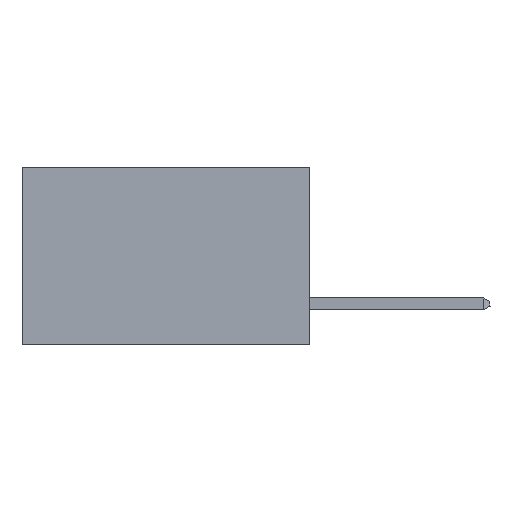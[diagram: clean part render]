
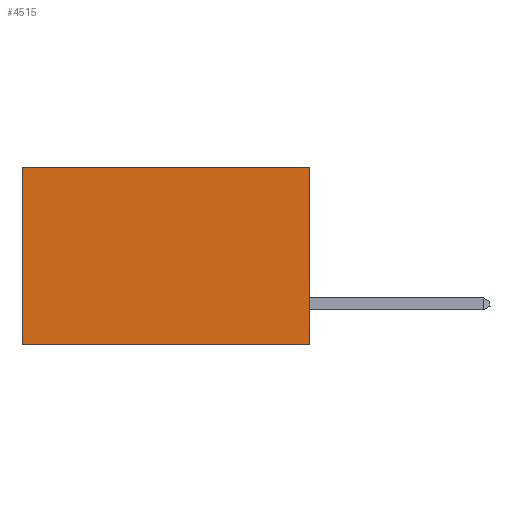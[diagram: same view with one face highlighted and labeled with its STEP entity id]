
A CAD part, left-side view. The second image highlights one B-rep face of the part: STEP entity #4515.
In plain terms, the highlighted planar face has unit normal (-1, 0, 0).
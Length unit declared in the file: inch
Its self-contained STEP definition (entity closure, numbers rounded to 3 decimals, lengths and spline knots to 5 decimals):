
#1781 = CARTESIAN_POINT ( 'NONE',  ( 0.2875, 0., -0.37 ) ) ;
#1880 = FACE_OUTER_BOUND ( 'NONE', #12481, .T. ) ;
#2175 = PLANE ( 'NONE',  #12967 ) ;
#2364 = EDGE_CURVE ( 'NONE', #7530, #5329, #20781, .T. ) ;
#2672 = EDGE_CURVE ( 'NONE', #15979, #6745, #7477, .T. ) ;
#4515 = ADVANCED_FACE ( 'NONE', ( #1880 ), #2175, .F. ) ;
#5237 = CARTESIAN_POINT ( 'NONE',  ( 0.2875, 0., 0. ) ) ;
#5238 = EDGE_CURVE ( 'NONE', #5329, #6745, #22425, .T. ) ;
#5329 = VERTEX_POINT ( 'NONE', #9780 ) ;
#5501 = VECTOR ( 'NONE', #18746, 39.37008 ) ;
#6745 = VERTEX_POINT ( 'NONE', #16134 ) ;
#7477 = LINE ( 'NONE', #1781, #21686 ) ;
#7530 = VERTEX_POINT ( 'NONE', #15555 ) ;
#7654 = DIRECTION ( 'NONE',  ( 0., 1., 0. ) ) ;
#7780 = ORIENTED_EDGE ( 'NONE', *, *, #2672, .F. ) ;
#9309 = CARTESIAN_POINT ( 'NONE',  ( 0.2875, 0.6, 0. ) ) ;
#9617 = ORIENTED_EDGE ( 'NONE', *, *, #5238, .T. ) ;
#9780 = CARTESIAN_POINT ( 'NONE',  ( 0.2875, 0.6, 0. ) ) ;
#9944 = DIRECTION ( 'NONE',  ( 0., 0., -1. ) ) ;
#10057 = ORIENTED_EDGE ( 'NONE', *, *, #12889, .F. ) ;
#12413 = CARTESIAN_POINT ( 'NONE',  ( 0.2875, 0., -0.37 ) ) ;
#12481 = EDGE_LOOP ( 'NONE', ( #9617, #7780, #10057, #22174 ) ) ;
#12889 = EDGE_CURVE ( 'NONE', #7530, #15979, #24249, .T. ) ;
#12928 = DIRECTION ( 'NONE',  ( 0., 1., 0. ) ) ;
#12967 = AXIS2_PLACEMENT_3D ( 'NONE', #13838, #21582, #17391 ) ;
#13838 = CARTESIAN_POINT ( 'NONE',  ( 0.2875, 0., 0. ) ) ;
#15555 = CARTESIAN_POINT ( 'NONE',  ( 0.2875, 0., 0. ) ) ;
#15979 = VERTEX_POINT ( 'NONE', #12413 ) ;
#16134 = CARTESIAN_POINT ( 'NONE',  ( 0.2875, 0.6, -0.37 ) ) ;
#17391 = DIRECTION ( 'NONE',  ( 0., 0., -1. ) ) ;
#18746 = DIRECTION ( 'NONE',  ( 0., 0., -1. ) ) ;
#20781 = LINE ( 'NONE', #5237, #23841 ) ;
#21544 = CARTESIAN_POINT ( 'NONE',  ( 0.2875, 0., 0. ) ) ;
#21582 = DIRECTION ( 'NONE',  ( 1., 0., 0. ) ) ;
#21686 = VECTOR ( 'NONE', #7654, 39.37008 ) ;
#22174 = ORIENTED_EDGE ( 'NONE', *, *, #2364, .T. ) ;
#22425 = LINE ( 'NONE', #9309, #5501 ) ;
#22713 = VECTOR ( 'NONE', #9944, 39.37008 ) ;
#23841 = VECTOR ( 'NONE', #12928, 39.37008 ) ;
#24249 = LINE ( 'NONE', #21544, #22713 ) ;
